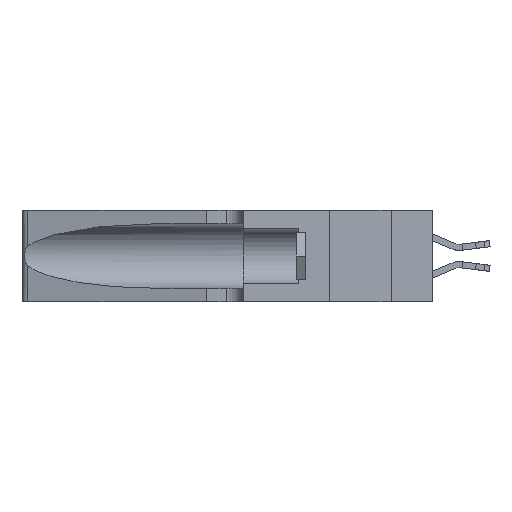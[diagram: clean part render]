
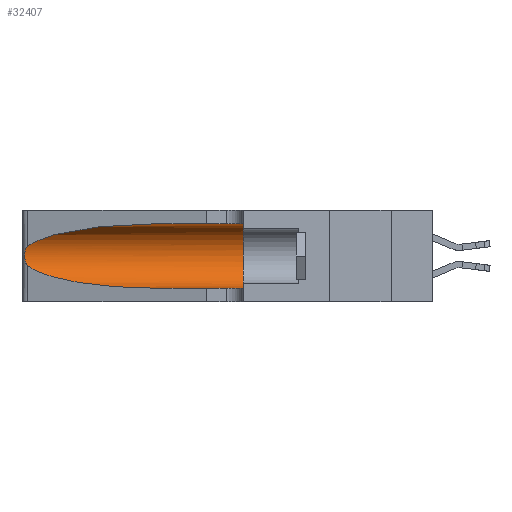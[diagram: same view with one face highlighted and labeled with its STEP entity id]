
A CAD part, left-side view. The second image highlights one B-rep face of the part: STEP entity #32407.
In plain terms, the highlighted cylindrical face has radius 3.308 mm (diameter 6.617 mm), a partial arc.
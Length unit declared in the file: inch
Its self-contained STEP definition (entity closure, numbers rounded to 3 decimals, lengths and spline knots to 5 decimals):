
#167 = CARTESIAN_POINT ( 'NONE',  ( 0.26017, 1.23833, 0.17102 ) ) ;
#234 = CARTESIAN_POINT ( 'NONE',  ( 0.1305, 1.61858, 0.185 ) ) ;
#333 = CARTESIAN_POINT ( 'NONE',  ( 0.1305, 0.72297, 0.31525 ) ) ;
#633 = ORIENTED_EDGE ( 'NONE', *, *, #6066, .F. ) ;
#852 = CARTESIAN_POINT ( 'NONE',  ( 0.1305, 0.35, 0.185 ) ) ;
#977 = VERTEX_POINT ( 'NONE', #12492 ) ;
#1126 = VERTEX_POINT ( 'NONE', #13872 ) ;
#2466 = CARTESIAN_POINT ( 'NONE',  ( 0.18966, 0.96281, 0.05475 ) ) ;
#2534 = CARTESIAN_POINT ( 'NONE',  ( 0.25487, 1.22718, 0.22369 ) ) ;
#2745 = CARTESIAN_POINT ( 'NONE',  ( 0.25789, 1.23486, 0.15765 ) ) ;
#3401 = CYLINDRICAL_SURFACE ( 'NONE', #12547, 0.13025 ) ;
#3424 = DIRECTION ( 'NONE',  ( 0., 0., 1. ) ) ;
#3452 = ORIENTED_EDGE ( 'NONE', *, *, #11367, .T. ) ;
#4730 = EDGE_CURVE ( 'NONE', #14989, #977, #18635, .T. ) ;
#4913 = CARTESIAN_POINT ( 'NONE',  ( 0.2373, 1.15595, 0.08982 ) ) ;
#5325 = CARTESIAN_POINT ( 'NONE',  ( 0.25555, 1.22993, 0.14849 ) ) ;
#5484 = CARTESIAN_POINT ( 'NONE',  ( 0.25487, 1.22718, 0.22369 ) ) ;
#6066 = EDGE_CURVE ( 'NONE', #977, #15983, #10923, .T. ) ;
#6244 = B_SPLINE_CURVE_WITH_KNOTS ( 'NONE', 3,
 ( #2534, #18010, #25638, #10374, #28143, #12949, #30702, #15558, #167, #18114, #2745, #20678, #5325, #23227 ),
 .UNSPECIFIED., .F., .F.,
 ( 4, 2, 2, 2, 2, 2, 4 ),
 ( 0., 0.00027, 0.00053, 0.00107, 0.0016, 0.00187, 0.00214 ),
 .UNSPECIFIED. ) ;
#8730 =( BOUNDED_CURVE ( )  B_SPLINE_CURVE ( 3, ( #333, #15714, #20829, #5484 ),
 .UNSPECIFIED., .F., .T. ) 
 B_SPLINE_CURVE_WITH_KNOTS ( ( 4, 4 ),
 ( 1.5708, 2.84003 ),
 .UNSPECIFIED. ) 
 CURVE ( )  GEOMETRIC_REPRESENTATION_ITEM ( )  RATIONAL_B_SPLINE_CURVE ( ( 1., 0.87, 0.87, 1. ) ) 
 REPRESENTATION_ITEM ( '' )  );
#9412 = ORIENTED_EDGE ( 'NONE', *, *, #20928, .T. ) ;
#10374 = CARTESIAN_POINT ( 'NONE',  ( 0.25787, 1.23484, 0.2124 ) ) ;
#10923 = CIRCLE ( 'NONE', #32740, 0.13025 ) ;
#11030 = FACE_OUTER_BOUND ( 'NONE', #13703, .T. ) ;
#11195 = VERTEX_POINT ( 'NONE', #28908 ) ;
#11367 = EDGE_CURVE ( 'NONE', #11195, #15983, #19382, .T. ) ;
#12034 = CARTESIAN_POINT ( 'NONE',  ( 0.25487, 1.22718, 0.14631 ) ) ;
#12492 = CARTESIAN_POINT ( 'NONE',  ( 0.1305, 0.35, 0.31525 ) ) ;
#12547 = AXIS2_PLACEMENT_3D ( 'NONE', #234, #20734, #13010 ) ;
#12949 = CARTESIAN_POINT ( 'NONE',  ( 0.26018, 1.23835, 0.19895 ) ) ;
#13010 = DIRECTION ( 'NONE',  ( 0., 0., -1. ) ) ;
#13367 = ORIENTED_EDGE ( 'NONE', *, *, #32811, .T. ) ;
#13703 = EDGE_LOOP ( 'NONE', ( #17591, #9412, #13367, #3452, #633, #21966 ) ) ;
#13872 = CARTESIAN_POINT ( 'NONE',  ( 0.25487, 1.22718, 0.22369 ) ) ;
#14286 = CARTESIAN_POINT ( 'NONE',  ( 0.1305, 1.61858, 0.05475 ) ) ;
#14827 = EDGE_CURVE ( 'NONE', #14989, #1126, #8730, .T. ) ;
#14989 = VERTEX_POINT ( 'NONE', #16455 ) ;
#15558 = CARTESIAN_POINT ( 'NONE',  ( 0.26075, 1.23896, 0.178 ) ) ;
#15714 = CARTESIAN_POINT ( 'NONE',  ( 0.18966, 0.96281, 0.31525 ) ) ;
#15983 = VERTEX_POINT ( 'NONE', #27673 ) ;
#16455 = CARTESIAN_POINT ( 'NONE',  ( 0.1305, 0.72297, 0.31525 ) ) ;
#17591 = ORIENTED_EDGE ( 'NONE', *, *, #14827, .T. ) ;
#18010 = CARTESIAN_POINT ( 'NONE',  ( 0.25555, 1.22994, 0.2215 ) ) ;
#18114 = CARTESIAN_POINT ( 'NONE',  ( 0.25856, 1.23593, 0.16098 ) ) ;
#18635 = LINE ( 'NONE', #31223, #31289 ) ;
#18778 = DIRECTION ( 'NONE',  ( 0., 1., 0. ) ) ;
#19382 = LINE ( 'NONE', #14286, #32017 ) ;
#20391 = CARTESIAN_POINT ( 'NONE',  ( 0.1305, 0.72297, 0.05475 ) ) ;
#20678 = CARTESIAN_POINT ( 'NONE',  ( 0.25639, 1.23186, 0.15144 ) ) ;
#20734 = DIRECTION ( 'NONE',  ( 0., -1., 0. ) ) ;
#20829 = CARTESIAN_POINT ( 'NONE',  ( 0.2373, 1.15595, 0.28018 ) ) ;
#20928 = EDGE_CURVE ( 'NONE', #1126, #21334, #6244, .T. ) ;
#21189 = DIRECTION ( 'NONE',  ( 0., -1., 0. ) ) ;
#21334 = VERTEX_POINT ( 'NONE', #12034 ) ;
#21966 = ORIENTED_EDGE ( 'NONE', *, *, #4730, .F. ) ;
#23227 = CARTESIAN_POINT ( 'NONE',  ( 0.25487, 1.22718, 0.14631 ) ) ;
#24509 = DIRECTION ( 'NONE',  ( 0., -1., 0. ) ) ;
#25088 =( BOUNDED_CURVE ( )  B_SPLINE_CURVE ( 3, ( #32959, #4913, #2466, #20391 ),
 .UNSPECIFIED., .F., .F. ) 
 B_SPLINE_CURVE_WITH_KNOTS ( ( 4, 4 ),
 ( 3.44316, 4.71239 ),
 .UNSPECIFIED. ) 
 CURVE ( )  GEOMETRIC_REPRESENTATION_ITEM ( )  RATIONAL_B_SPLINE_CURVE ( ( 1., 0.87, 0.87, 1. ) ) 
 REPRESENTATION_ITEM ( '' )  );
#25638 = CARTESIAN_POINT ( 'NONE',  ( 0.25639, 1.23184, 0.21858 ) ) ;
#27673 = CARTESIAN_POINT ( 'NONE',  ( 0.1305, 0.35, 0.05475 ) ) ;
#28143 = CARTESIAN_POINT ( 'NONE',  ( 0.25854, 1.2359, 0.20912 ) ) ;
#28908 = CARTESIAN_POINT ( 'NONE',  ( 0.1305, 0.72297, 0.05475 ) ) ;
#30702 = CARTESIAN_POINT ( 'NONE',  ( 0.26075, 1.23896, 0.19203 ) ) ;
#31223 = CARTESIAN_POINT ( 'NONE',  ( 0.1305, 1.61858, 0.31525 ) ) ;
#31289 = VECTOR ( 'NONE', #21189, 39.37008 ) ;
#32017 = VECTOR ( 'NONE', #24509, 39.37008 ) ;
#32407 = ADVANCED_FACE ( 'NONE', ( #11030 ), #3401, .F. ) ;
#32740 = AXIS2_PLACEMENT_3D ( 'NONE', #852, #18778, #3424 ) ;
#32811 = EDGE_CURVE ( 'NONE', #21334, #11195, #25088, .T. ) ;
#32959 = CARTESIAN_POINT ( 'NONE',  ( 0.25487, 1.22718, 0.14631 ) ) ;
